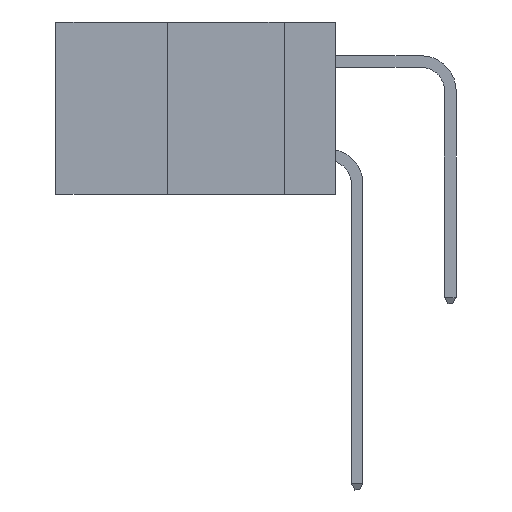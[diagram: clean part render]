
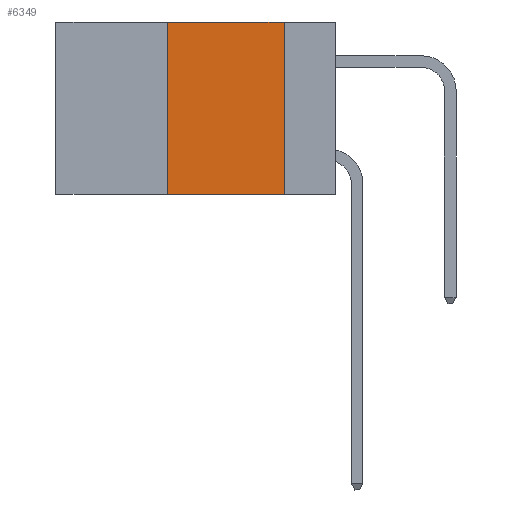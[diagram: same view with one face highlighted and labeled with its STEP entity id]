
A CAD part, left-side view. The second image highlights one B-rep face of the part: STEP entity #6349.
In plain terms, the highlighted planar face has unit normal (-1, 0, 0).
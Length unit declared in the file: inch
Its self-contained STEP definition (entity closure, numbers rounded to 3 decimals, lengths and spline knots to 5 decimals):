
#213 = DIRECTION ( 'NONE',  ( 0., 0., -1. ) ) ;
#383 = DIRECTION ( 'NONE',  ( 0., 0., 1. ) ) ;
#761 = VERTEX_POINT ( 'NONE', #3382 ) ;
#1254 = CARTESIAN_POINT ( 'NONE',  ( 0., 0.6, 0. ) ) ;
#2493 = DIRECTION ( 'NONE',  ( 0., 0., -1. ) ) ;
#2586 = EDGE_CURVE ( 'NONE', #10803, #13687, #3468, .T. ) ;
#2718 = VECTOR ( 'NONE', #383, 39.37008 ) ;
#2858 = CARTESIAN_POINT ( 'NONE',  ( 0., 0.6, -0.37 ) ) ;
#3068 = VECTOR ( 'NONE', #213, 39.37008 ) ;
#3382 = CARTESIAN_POINT ( 'NONE',  ( 0., 0.11, -0.37 ) ) ;
#3457 = LINE ( 'NONE', #5931, #3068 ) ;
#3468 = LINE ( 'NONE', #6236, #5903 ) ;
#3638 = EDGE_CURVE ( 'NONE', #13687, #761, #3457, .T. ) ;
#3680 = EDGE_CURVE ( 'NONE', #8255, #10803, #4974, .T. ) ;
#3684 = EDGE_CURVE ( 'NONE', #8255, #761, #7613, .T. ) ;
#4974 = LINE ( 'NONE', #7064, #2718 ) ;
#5903 = VECTOR ( 'NONE', #11344, 39.37008 ) ;
#5931 = CARTESIAN_POINT ( 'NONE',  ( 0., 0.11, 0. ) ) ;
#5981 = CARTESIAN_POINT ( 'NONE',  ( 0., 0.11, 0. ) ) ;
#6236 = CARTESIAN_POINT ( 'NONE',  ( 0., 0.6, 0. ) ) ;
#6349 = ADVANCED_FACE ( 'NONE', ( #7383 ), #7728, .F. ) ;
#6913 = ORIENTED_EDGE ( 'NONE', *, *, #3638, .F. ) ;
#7064 = CARTESIAN_POINT ( 'NONE',  ( 0., 0.36, 0. ) ) ;
#7383 = FACE_OUTER_BOUND ( 'NONE', #12619, .T. ) ;
#7613 = LINE ( 'NONE', #2858, #10020 ) ;
#7728 = PLANE ( 'NONE',  #11504 ) ;
#7742 = ORIENTED_EDGE ( 'NONE', *, *, #3680, .F. ) ;
#7752 = ORIENTED_EDGE ( 'NONE', *, *, #3684, .T. ) ;
#7973 = ORIENTED_EDGE ( 'NONE', *, *, #2586, .F. ) ;
#8255 = VERTEX_POINT ( 'NONE', #11807 ) ;
#8748 = DIRECTION ( 'NONE',  ( 1., 0., 0. ) ) ;
#9100 = DIRECTION ( 'NONE',  ( 0., -1., 0. ) ) ;
#9924 = CARTESIAN_POINT ( 'NONE',  ( 0., 0.36, 0. ) ) ;
#10020 = VECTOR ( 'NONE', #9100, 39.37008 ) ;
#10803 = VERTEX_POINT ( 'NONE', #9924 ) ;
#11344 = DIRECTION ( 'NONE',  ( 0., -1., 0. ) ) ;
#11504 = AXIS2_PLACEMENT_3D ( 'NONE', #1254, #8748, #2493 ) ;
#11807 = CARTESIAN_POINT ( 'NONE',  ( 0., 0.36, -0.37 ) ) ;
#12619 = EDGE_LOOP ( 'NONE', ( #6913, #7973, #7742, #7752 ) ) ;
#13687 = VERTEX_POINT ( 'NONE', #5981 ) ;
